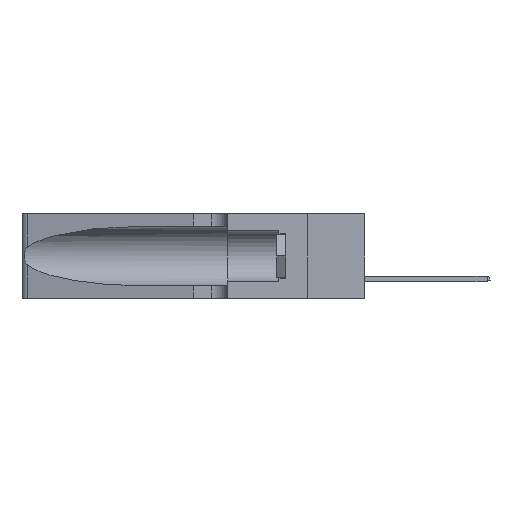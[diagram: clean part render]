
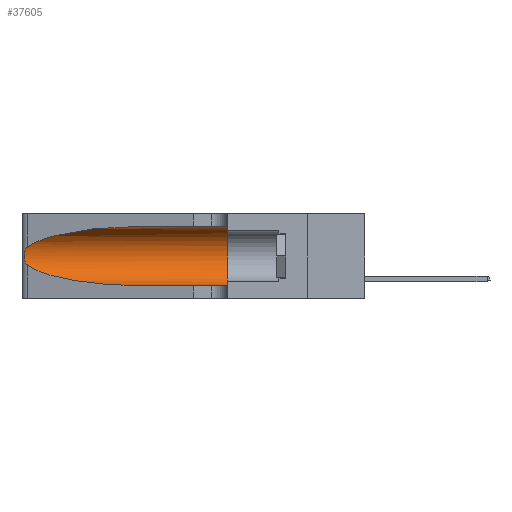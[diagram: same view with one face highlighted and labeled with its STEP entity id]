
A CAD part, left-side view. The second image highlights one B-rep face of the part: STEP entity #37605.
In plain terms, the highlighted cylindrical face has radius 3.308 mm (diameter 6.617 mm), a partial arc.
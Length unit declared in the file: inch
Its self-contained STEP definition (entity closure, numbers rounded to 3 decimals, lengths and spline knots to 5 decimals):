
#142 = CYLINDRICAL_SURFACE ( 'NONE', #37229, 0.13025 ) ;
#2093 = DIRECTION ( 'NONE',  ( 0., 1., 0. ) ) ;
#3163 = CARTESIAN_POINT ( 'NONE',  ( 0.25487, 1.22718, 0.14631 ) ) ;
#3244 = EDGE_CURVE ( 'NONE', #18993, #16842, #23209, .T. ) ;
#3720 = ORIENTED_EDGE ( 'NONE', *, *, #33319, .T. ) ;
#3917 = CARTESIAN_POINT ( 'NONE',  ( 0.2373, 1.15595, 0.08982 ) ) ;
#4894 = CARTESIAN_POINT ( 'NONE',  ( 0.1305, 0.72297, 0.05475 ) ) ;
#5350 = CARTESIAN_POINT ( 'NONE',  ( 0.25639, 1.23184, 0.21858 ) ) ;
#5969 = CARTESIAN_POINT ( 'NONE',  ( 0.1305, 1.61858, 0.31525 ) ) ;
#6259 = DIRECTION ( 'NONE',  ( 0., 0., 1. ) ) ;
#6488 = CARTESIAN_POINT ( 'NONE',  ( 0.1305, 0.35, 0.31525 ) ) ;
#6591 = ORIENTED_EDGE ( 'NONE', *, *, #13971, .T. ) ;
#8332 =( BOUNDED_CURVE ( )  B_SPLINE_CURVE ( 3, ( #34614, #12704, #9697, #20651 ),
 .UNSPECIFIED., .F., .T. ) 
 B_SPLINE_CURVE_WITH_KNOTS ( ( 4, 4 ),
 ( 1.5708, 2.84003 ),
 .UNSPECIFIED. ) 
 CURVE ( )  GEOMETRIC_REPRESENTATION_ITEM ( )  RATIONAL_B_SPLINE_CURVE ( ( 1., 0.87, 0.87, 1. ) ) 
 REPRESENTATION_ITEM ( '' )  );
#8758 = VERTEX_POINT ( 'NONE', #24669 ) ;
#8860 = VECTOR ( 'NONE', #16005, 39.37008 ) ;
#8879 = CARTESIAN_POINT ( 'NONE',  ( 0.1305, 1.61858, 0.05475 ) ) ;
#9697 = CARTESIAN_POINT ( 'NONE',  ( 0.2373, 1.15595, 0.28018 ) ) ;
#10203 = CARTESIAN_POINT ( 'NONE',  ( 0.25789, 1.23486, 0.15765 ) ) ;
#10367 = CARTESIAN_POINT ( 'NONE',  ( 0.25856, 1.23593, 0.16098 ) ) ;
#11588 = VERTEX_POINT ( 'NONE', #39135 ) ;
#11832 = VECTOR ( 'NONE', #14801, 39.37008 ) ;
#11868 = VERTEX_POINT ( 'NONE', #26476 ) ;
#11873 = ORIENTED_EDGE ( 'NONE', *, *, #39382, .F. ) ;
#11906 = CIRCLE ( 'NONE', #44922, 0.13025 ) ;
#12580 = CARTESIAN_POINT ( 'NONE',  ( 0.25487, 1.22718, 0.22369 ) ) ;
#12704 = CARTESIAN_POINT ( 'NONE',  ( 0.18966, 0.96281, 0.31525 ) ) ;
#13676 = LINE ( 'NONE', #8879, #8860 ) ;
#13854 = CARTESIAN_POINT ( 'NONE',  ( 0.26075, 1.23896, 0.178 ) ) ;
#13971 = EDGE_CURVE ( 'NONE', #16842, #11588, #38564, .T. ) ;
#14426 = DIRECTION ( 'NONE',  ( 0., 0., -1. ) ) ;
#14662 = EDGE_LOOP ( 'NONE', ( #3720, #37627, #6591, #26600, #31731, #11873 ) ) ;
#14801 = DIRECTION ( 'NONE',  ( 0., -1., 0. ) ) ;
#16005 = DIRECTION ( 'NONE',  ( 0., -1., 0. ) ) ;
#16842 = VERTEX_POINT ( 'NONE', #3163 ) ;
#16989 = CARTESIAN_POINT ( 'NONE',  ( 0.25787, 1.23484, 0.2124 ) ) ;
#17162 = CARTESIAN_POINT ( 'NONE',  ( 0.26018, 1.23835, 0.19895 ) ) ;
#17691 = CARTESIAN_POINT ( 'NONE',  ( 0.25639, 1.23186, 0.15144 ) ) ;
#17920 = EDGE_CURVE ( 'NONE', #25242, #11868, #11906, .T. ) ;
#18190 = CARTESIAN_POINT ( 'NONE',  ( 0.25555, 1.22993, 0.14849 ) ) ;
#18993 = VERTEX_POINT ( 'NONE', #12580 ) ;
#20651 = CARTESIAN_POINT ( 'NONE',  ( 0.25487, 1.22718, 0.22369 ) ) ;
#22728 = CARTESIAN_POINT ( 'NONE',  ( 0.25487, 1.22718, 0.14631 ) ) ;
#23209 = B_SPLINE_CURVE_WITH_KNOTS ( 'NONE', 3,
 ( #32104, #24253, #5350, #16989, #39990, #17162, #36645, #13854, #48271, #10367, #10203, #17691, #18190, #33624 ),
 .UNSPECIFIED., .F., .F.,
 ( 4, 2, 2, 2, 2, 2, 4 ),
 ( 0., 0.00027, 0.00053, 0.00107, 0.0016, 0.00187, 0.00214 ),
 .UNSPECIFIED. ) ;
#24253 = CARTESIAN_POINT ( 'NONE',  ( 0.25555, 1.22994, 0.2215 ) ) ;
#24478 = FACE_OUTER_BOUND ( 'NONE', #14662, .T. ) ;
#24669 = CARTESIAN_POINT ( 'NONE',  ( 0.1305, 0.72297, 0.31525 ) ) ;
#25242 = VERTEX_POINT ( 'NONE', #6488 ) ;
#26476 = CARTESIAN_POINT ( 'NONE',  ( 0.1305, 0.35, 0.05475 ) ) ;
#26600 = ORIENTED_EDGE ( 'NONE', *, *, #28963, .T. ) ;
#28963 = EDGE_CURVE ( 'NONE', #11588, #11868, #13676, .T. ) ;
#28977 = CARTESIAN_POINT ( 'NONE',  ( 0.1305, 0.35, 0.185 ) ) ;
#31648 = CARTESIAN_POINT ( 'NONE',  ( 0.18966, 0.96281, 0.05475 ) ) ;
#31731 = ORIENTED_EDGE ( 'NONE', *, *, #17920, .F. ) ;
#32104 = CARTESIAN_POINT ( 'NONE',  ( 0.25487, 1.22718, 0.22369 ) ) ;
#33319 = EDGE_CURVE ( 'NONE', #8758, #18993, #8332, .T. ) ;
#33624 = CARTESIAN_POINT ( 'NONE',  ( 0.25487, 1.22718, 0.14631 ) ) ;
#34614 = CARTESIAN_POINT ( 'NONE',  ( 0.1305, 0.72297, 0.31525 ) ) ;
#36645 = CARTESIAN_POINT ( 'NONE',  ( 0.26075, 1.23896, 0.19203 ) ) ;
#37229 = AXIS2_PLACEMENT_3D ( 'NONE', #48368, #48692, #14426 ) ;
#37605 = ADVANCED_FACE ( 'NONE', ( #24478 ), #142, .F. ) ;
#37627 = ORIENTED_EDGE ( 'NONE', *, *, #3244, .T. ) ;
#38564 =( BOUNDED_CURVE ( )  B_SPLINE_CURVE ( 3, ( #22728, #3917, #31648, #4894 ),
 .UNSPECIFIED., .F., .F. ) 
 B_SPLINE_CURVE_WITH_KNOTS ( ( 4, 4 ),
 ( 3.44316, 4.71239 ),
 .UNSPECIFIED. ) 
 CURVE ( )  GEOMETRIC_REPRESENTATION_ITEM ( )  RATIONAL_B_SPLINE_CURVE ( ( 1., 0.87, 0.87, 1. ) ) 
 REPRESENTATION_ITEM ( '' )  );
#39135 = CARTESIAN_POINT ( 'NONE',  ( 0.1305, 0.72297, 0.05475 ) ) ;
#39382 = EDGE_CURVE ( 'NONE', #8758, #25242, #48220, .T. ) ;
#39990 = CARTESIAN_POINT ( 'NONE',  ( 0.25854, 1.2359, 0.20912 ) ) ;
#44922 = AXIS2_PLACEMENT_3D ( 'NONE', #28977, #2093, #6259 ) ;
#48220 = LINE ( 'NONE', #5969, #11832 ) ;
#48271 = CARTESIAN_POINT ( 'NONE',  ( 0.26017, 1.23833, 0.17102 ) ) ;
#48368 = CARTESIAN_POINT ( 'NONE',  ( 0.1305, 1.61858, 0.185 ) ) ;
#48692 = DIRECTION ( 'NONE',  ( 0., -1., 0. ) ) ;
